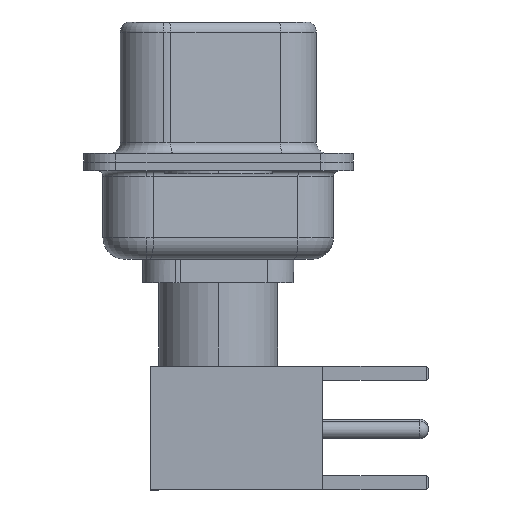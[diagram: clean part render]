
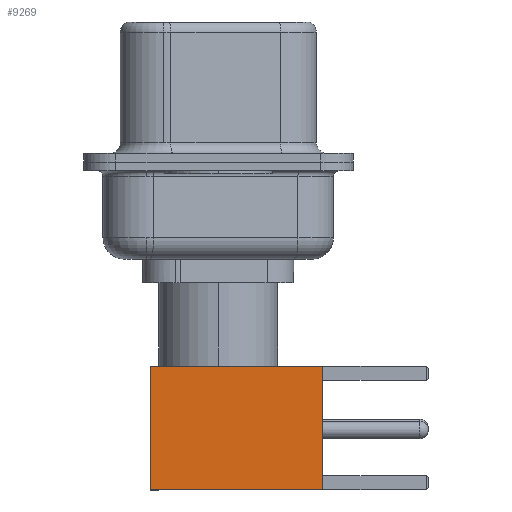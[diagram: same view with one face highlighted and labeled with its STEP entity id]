
A CAD part, left-side view. The second image highlights one B-rep face of the part: STEP entity #9269.
In plain terms, the highlighted face is planar.
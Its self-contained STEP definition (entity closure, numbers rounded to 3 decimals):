
#193 = VERTEX_POINT ( 'NONE', #5690 ) ;
#293 = VECTOR ( 'NONE', #15360, 1000. ) ;
#1597 = CARTESIAN_POINT ( 'NONE',  ( 2.875, 2.875, 0. ) ) ;
#2206 = EDGE_CURVE ( 'NONE', #6414, #193, #6012, .T. ) ;
#2700 = DIRECTION ( 'NONE',  ( 0., 0., -1. ) ) ;
#3115 = CARTESIAN_POINT ( 'NONE',  ( 2.875, 2.875, 0. ) ) ;
#3345 = DIRECTION ( 'NONE',  ( 0., 0., -1. ) ) ;
#3446 = VECTOR ( 'NONE', #2700, 1000. ) ;
#3591 = VERTEX_POINT ( 'NONE', #12502 ) ;
#5690 = CARTESIAN_POINT ( 'NONE',  ( -2.875, 2.875, 0. ) ) ;
#6012 = LINE ( 'NONE', #15577, #16626 ) ;
#6414 = VERTEX_POINT ( 'NONE', #17125 ) ;
#6903 = LINE ( 'NONE', #1597, #3446 ) ;
#7133 = LINE ( 'NONE', #14119, #293 ) ;
#7371 = AXIS2_PLACEMENT_3D ( 'NONE', #13012, #9145, #14690 ) ;
#7715 = FACE_OUTER_BOUND ( 'NONE', #16737, .T. ) ;
#8188 = ORIENTED_EDGE ( 'NONE', *, *, #2206, .F. ) ;
#8658 = EDGE_CURVE ( 'NONE', #3591, #6414, #14419, .T. ) ;
#9145 = DIRECTION ( 'NONE',  ( 0., 1., 0. ) ) ;
#9269 = ADVANCED_FACE ( 'NONE', ( #7715 ), #13100, .T. ) ;
#9841 = ORIENTED_EDGE ( 'NONE', *, *, #8658, .F. ) ;
#10124 = CARTESIAN_POINT ( 'NONE',  ( 0., 2.875, 8. ) ) ;
#11211 = EDGE_CURVE ( 'NONE', #3591, #11908, #6903, .T. ) ;
#11908 = VERTEX_POINT ( 'NONE', #3115 ) ;
#12502 = CARTESIAN_POINT ( 'NONE',  ( 2.875, 2.875, 8. ) ) ;
#13012 = CARTESIAN_POINT ( 'NONE',  ( 2.875, 2.875, 0. ) ) ;
#13100 = PLANE ( 'NONE',  #7371 ) ;
#13135 = EDGE_CURVE ( 'NONE', #11908, #193, #7133, .T. ) ;
#14119 = CARTESIAN_POINT ( 'NONE',  ( 0., 2.875, 0. ) ) ;
#14236 = ORIENTED_EDGE ( 'NONE', *, *, #11211, .T. ) ;
#14419 = LINE ( 'NONE', #10124, #16494 ) ;
#14690 = DIRECTION ( 'NONE',  ( 0., 0., 1. ) ) ;
#15360 = DIRECTION ( 'NONE',  ( -1., 0., 0. ) ) ;
#15577 = CARTESIAN_POINT ( 'NONE',  ( -2.875, 2.875, 0. ) ) ;
#15830 = DIRECTION ( 'NONE',  ( -1., 0., 0. ) ) ;
#16494 = VECTOR ( 'NONE', #15830, 1000. ) ;
#16626 = VECTOR ( 'NONE', #3345, 1000. ) ;
#16708 = ORIENTED_EDGE ( 'NONE', *, *, #13135, .T. ) ;
#16737 = EDGE_LOOP ( 'NONE', ( #14236, #16708, #8188, #9841 ) ) ;
#17125 = CARTESIAN_POINT ( 'NONE',  ( -2.875, 2.875, 8. ) ) ;
